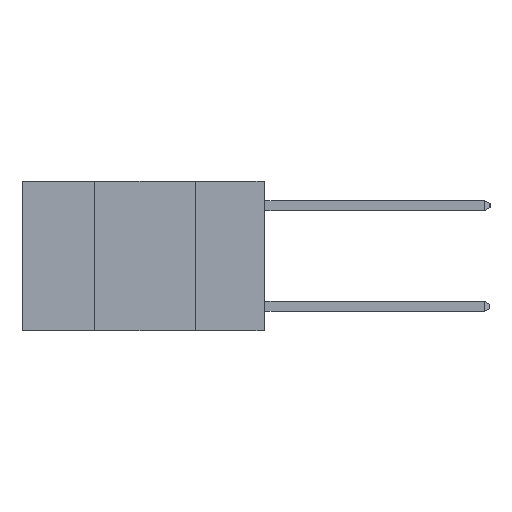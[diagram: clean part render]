
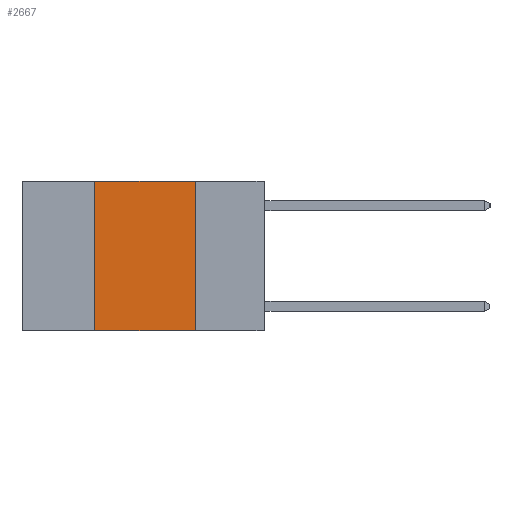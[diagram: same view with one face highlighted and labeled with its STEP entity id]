
A CAD part, left-side view. The second image highlights one B-rep face of the part: STEP entity #2667.
In plain terms, the highlighted planar face has unit normal (-1, 0, 0).
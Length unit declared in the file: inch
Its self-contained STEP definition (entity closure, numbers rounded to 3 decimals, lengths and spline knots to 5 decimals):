
#20 = ORIENTED_EDGE ( 'NONE', *, *, #7872, .F. ) ;
#46 = DIRECTION ( 'NONE',  ( 0., 0., -1. ) ) ;
#105 = CARTESIAN_POINT ( 'NONE',  ( 0., 0.17, 0. ) ) ;
#225 = CARTESIAN_POINT ( 'NONE',  ( 0., 0.42, -0.37 ) ) ;
#261 = FACE_OUTER_BOUND ( 'NONE', #5436, .T. ) ;
#718 = ORIENTED_EDGE ( 'NONE', *, *, #3893, .F. ) ;
#719 = CARTESIAN_POINT ( 'NONE',  ( 0., 0.42, 0. ) ) ;
#1075 = VERTEX_POINT ( 'NONE', #1372 ) ;
#1372 = CARTESIAN_POINT ( 'NONE',  ( 0., 0.17, -0.37 ) ) ;
#1481 = ORIENTED_EDGE ( 'NONE', *, *, #5625, .T. ) ;
#1830 = CARTESIAN_POINT ( 'NONE',  ( 0., 0.17, 0. ) ) ;
#2119 = VECTOR ( 'NONE', #2120, 39.37008 ) ;
#2120 = DIRECTION ( 'NONE',  ( 0., 0., 1. ) ) ;
#2155 = LINE ( 'NONE', #5506, #2119 ) ;
#2424 = VECTOR ( 'NONE', #6739, 39.37008 ) ;
#2507 = LINE ( 'NONE', #6804, #2424 ) ;
#2551 = VECTOR ( 'NONE', #46, 39.37008 ) ;
#2567 = LINE ( 'NONE', #105, #2551 ) ;
#2667 = ADVANCED_FACE ( 'NONE', ( #261 ), #3189, .F. ) ;
#2797 = DIRECTION ( 'NONE',  ( 0., 0., -1. ) ) ;
#2851 = DIRECTION ( 'NONE',  ( 1., 0., 0. ) ) ;
#3189 = PLANE ( 'NONE',  #6848 ) ;
#3893 = EDGE_CURVE ( 'NONE', #4663, #7595, #2507, .T. ) ;
#4663 = VERTEX_POINT ( 'NONE', #719 ) ;
#4730 = CARTESIAN_POINT ( 'NONE',  ( 0., 0.6, 0. ) ) ;
#4759 = VERTEX_POINT ( 'NONE', #225 ) ;
#5067 = ORIENTED_EDGE ( 'NONE', *, *, #8123, .F. ) ;
#5436 = EDGE_LOOP ( 'NONE', ( #20, #718, #5067, #1481 ) ) ;
#5506 = CARTESIAN_POINT ( 'NONE',  ( 0., 0.42, 0. ) ) ;
#5625 = EDGE_CURVE ( 'NONE', #4759, #1075, #6933, .T. ) ;
#6739 = DIRECTION ( 'NONE',  ( 0., -1., 0. ) ) ;
#6804 = CARTESIAN_POINT ( 'NONE',  ( 0., 0.6, 0. ) ) ;
#6848 = AXIS2_PLACEMENT_3D ( 'NONE', #4730, #2851, #2797 ) ;
#6880 = VECTOR ( 'NONE', #7316, 39.37008 ) ;
#6933 = LINE ( 'NONE', #7425, #6880 ) ;
#7316 = DIRECTION ( 'NONE',  ( 0., -1., 0. ) ) ;
#7425 = CARTESIAN_POINT ( 'NONE',  ( 0., 0.6, -0.37 ) ) ;
#7595 = VERTEX_POINT ( 'NONE', #1830 ) ;
#7872 = EDGE_CURVE ( 'NONE', #7595, #1075, #2567, .T. ) ;
#8123 = EDGE_CURVE ( 'NONE', #4759, #4663, #2155, .T. ) ;
